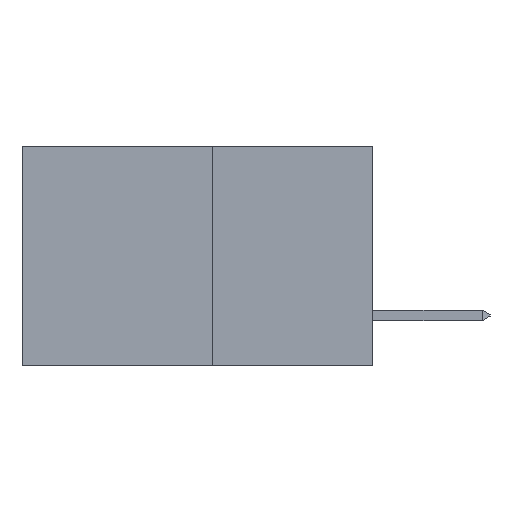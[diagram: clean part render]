
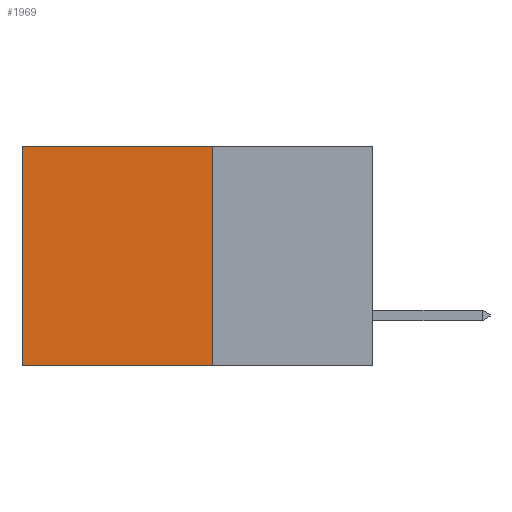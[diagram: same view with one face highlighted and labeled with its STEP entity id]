
A CAD part, left-side view. The second image highlights one B-rep face of the part: STEP entity #1969.
In plain terms, the highlighted planar face has unit normal (-1, 0, 0).
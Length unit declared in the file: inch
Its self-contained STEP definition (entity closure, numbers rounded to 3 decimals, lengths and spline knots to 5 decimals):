
#373 = DIRECTION ( 'NONE',  ( 0., 1., 0. ) ) ;
#1151 = FACE_OUTER_BOUND ( 'NONE', #4015, .T. ) ;
#1547 = VECTOR ( 'NONE', #14080, 39.37008 ) ;
#1969 = ADVANCED_FACE ( 'NONE', ( #1151 ), #18234, .F. ) ;
#2170 = EDGE_CURVE ( 'NONE', #20835, #12201, #18189, .T. ) ;
#2393 = ORIENTED_EDGE ( 'NONE', *, *, #11524, .F. ) ;
#4015 = EDGE_LOOP ( 'NONE', ( #11210, #2393, #20748, #10961 ) ) ;
#4284 = VECTOR ( 'NONE', #21458, 39.37008 ) ;
#4443 = EDGE_CURVE ( 'NONE', #11497, #20625, #21545, .T. ) ;
#5345 = CARTESIAN_POINT ( 'NONE',  ( 0.277, 0.27, -0.37 ) ) ;
#5946 = LINE ( 'NONE', #10687, #16421 ) ;
#7119 = LINE ( 'NONE', #22780, #1547 ) ;
#8052 = CARTESIAN_POINT ( 'NONE',  ( 0.277, 0.59, 0. ) ) ;
#8445 = DIRECTION ( 'NONE',  ( 0., 0., -1. ) ) ;
#8548 = CARTESIAN_POINT ( 'NONE',  ( 0.277, 0.59, -0.37 ) ) ;
#10687 = CARTESIAN_POINT ( 'NONE',  ( 0.277, 0.27, 0. ) ) ;
#10961 = ORIENTED_EDGE ( 'NONE', *, *, #23057, .T. ) ;
#11210 = ORIENTED_EDGE ( 'NONE', *, *, #2170, .T. ) ;
#11497 = VERTEX_POINT ( 'NONE', #18733 ) ;
#11524 = EDGE_CURVE ( 'NONE', #20625, #12201, #7119, .T. ) ;
#12201 = VERTEX_POINT ( 'NONE', #14427 ) ;
#12614 = VECTOR ( 'NONE', #8445, 39.37008 ) ;
#14080 = DIRECTION ( 'NONE',  ( 0., 1., 0. ) ) ;
#14427 = CARTESIAN_POINT ( 'NONE',  ( 0.277, 0.59, -0.37 ) ) ;
#16127 = AXIS2_PLACEMENT_3D ( 'NONE', #18038, #17765, #17520 ) ;
#16421 = VECTOR ( 'NONE', #373, 39.37008 ) ;
#17520 = DIRECTION ( 'NONE',  ( 0., 0., -1. ) ) ;
#17765 = DIRECTION ( 'NONE',  ( 1., 0., 0. ) ) ;
#18038 = CARTESIAN_POINT ( 'NONE',  ( 0.277, 0.27, -0.37 ) ) ;
#18189 = LINE ( 'NONE', #8548, #12614 ) ;
#18234 = PLANE ( 'NONE',  #16127 ) ;
#18733 = CARTESIAN_POINT ( 'NONE',  ( 0.277, 0.27, 0. ) ) ;
#20625 = VERTEX_POINT ( 'NONE', #5345 ) ;
#20748 = ORIENTED_EDGE ( 'NONE', *, *, #4443, .F. ) ;
#20835 = VERTEX_POINT ( 'NONE', #8052 ) ;
#21458 = DIRECTION ( 'NONE',  ( 0., 0., -1. ) ) ;
#21545 = LINE ( 'NONE', #21597, #4284 ) ;
#21597 = CARTESIAN_POINT ( 'NONE',  ( 0.277, 0.27, -0.37 ) ) ;
#22780 = CARTESIAN_POINT ( 'NONE',  ( 0.277, 0.27, -0.37 ) ) ;
#23057 = EDGE_CURVE ( 'NONE', #11497, #20835, #5946, .T. ) ;
